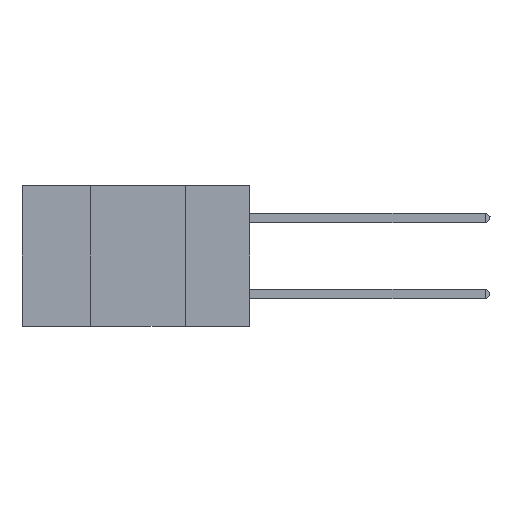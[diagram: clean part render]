
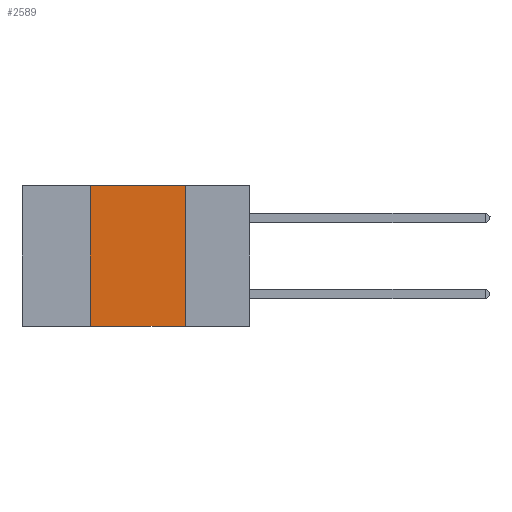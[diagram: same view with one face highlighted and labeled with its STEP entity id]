
A CAD part, left-side view. The second image highlights one B-rep face of the part: STEP entity #2589.
In plain terms, the highlighted planar face has unit normal (-1, 0, 0).
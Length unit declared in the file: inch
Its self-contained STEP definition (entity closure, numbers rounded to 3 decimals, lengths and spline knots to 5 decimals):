
#434 = ORIENTED_EDGE ( 'NONE', *, *, #3365, .F. ) ;
#814 = VERTEX_POINT ( 'NONE', #6159 ) ;
#938 = VECTOR ( 'NONE', #6483, 39.37008 ) ;
#1091 = AXIS2_PLACEMENT_3D ( 'NONE', #8502, #3299, #4740 ) ;
#1154 = FACE_OUTER_BOUND ( 'NONE', #1493, .T. ) ;
#1493 = EDGE_LOOP ( 'NONE', ( #1617, #434, #6053, #3755 ) ) ;
#1617 = ORIENTED_EDGE ( 'NONE', *, *, #1803, .F. ) ;
#1796 = VERTEX_POINT ( 'NONE', #5006 ) ;
#1797 = DIRECTION ( 'NONE',  ( 0., -1., 0. ) ) ;
#1803 = EDGE_CURVE ( 'NONE', #9292, #814, #6391, .T. ) ;
#1999 = CARTESIAN_POINT ( 'NONE',  ( 0., 0.17, 0. ) ) ;
#2451 = CARTESIAN_POINT ( 'NONE',  ( 0., 0.42, -0.37 ) ) ;
#2588 = VECTOR ( 'NONE', #1797, 39.37008 ) ;
#2589 = ADVANCED_FACE ( 'NONE', ( #1154 ), #8548, .F. ) ;
#2902 = VERTEX_POINT ( 'NONE', #2451 ) ;
#3299 = DIRECTION ( 'NONE',  ( 1., 0., 0. ) ) ;
#3365 = EDGE_CURVE ( 'NONE', #1796, #9292, #5931, .T. ) ;
#3546 = CARTESIAN_POINT ( 'NONE',  ( 0., 0.17, 0. ) ) ;
#3755 = ORIENTED_EDGE ( 'NONE', *, *, #7157, .T. ) ;
#3797 = EDGE_CURVE ( 'NONE', #2902, #1796, #7733, .T. ) ;
#4740 = DIRECTION ( 'NONE',  ( 0., 0., -1. ) ) ;
#4900 = VECTOR ( 'NONE', #6368, 39.37008 ) ;
#5006 = CARTESIAN_POINT ( 'NONE',  ( 0., 0.42, 0. ) ) ;
#5704 = CARTESIAN_POINT ( 'NONE',  ( 0., 0.42, 0. ) ) ;
#5931 = LINE ( 'NONE', #8350, #6421 ) ;
#6053 = ORIENTED_EDGE ( 'NONE', *, *, #3797, .F. ) ;
#6159 = CARTESIAN_POINT ( 'NONE',  ( 0., 0.17, -0.37 ) ) ;
#6241 = LINE ( 'NONE', #9086, #2588 ) ;
#6368 = DIRECTION ( 'NONE',  ( 0., 0., 1. ) ) ;
#6391 = LINE ( 'NONE', #1999, #938 ) ;
#6421 = VECTOR ( 'NONE', #8208, 39.37008 ) ;
#6483 = DIRECTION ( 'NONE',  ( 0., 0., -1. ) ) ;
#7157 = EDGE_CURVE ( 'NONE', #2902, #814, #6241, .T. ) ;
#7733 = LINE ( 'NONE', #5704, #4900 ) ;
#8208 = DIRECTION ( 'NONE',  ( 0., -1., 0. ) ) ;
#8350 = CARTESIAN_POINT ( 'NONE',  ( 0., 0.6, 0. ) ) ;
#8502 = CARTESIAN_POINT ( 'NONE',  ( 0., 0.6, 0. ) ) ;
#8548 = PLANE ( 'NONE',  #1091 ) ;
#9086 = CARTESIAN_POINT ( 'NONE',  ( 0., 0.6, -0.37 ) ) ;
#9292 = VERTEX_POINT ( 'NONE', #3546 ) ;
